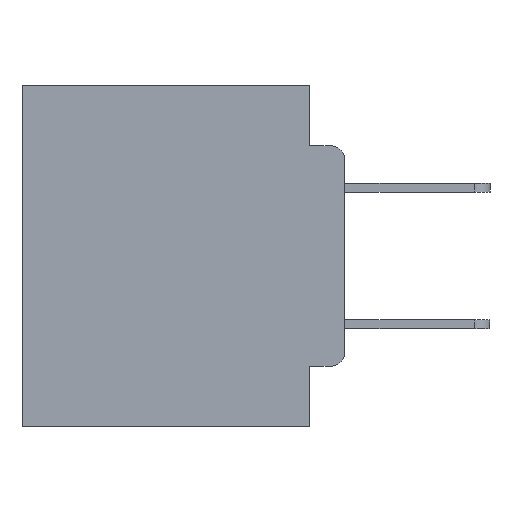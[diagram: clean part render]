
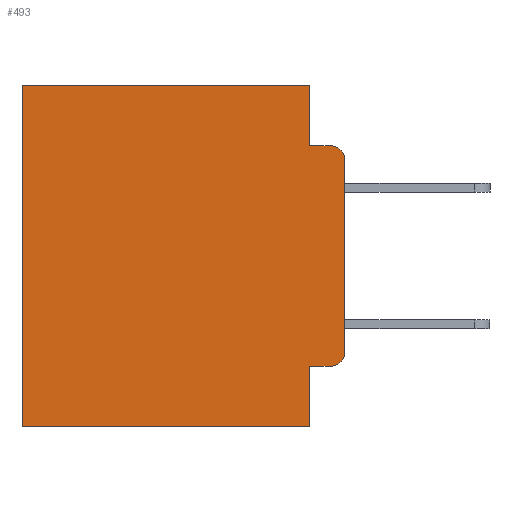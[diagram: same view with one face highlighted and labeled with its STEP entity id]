
A CAD part, left-side view. The second image highlights one B-rep face of the part: STEP entity #493.
In plain terms, the highlighted planar face has unit normal (-1, 0, 0).
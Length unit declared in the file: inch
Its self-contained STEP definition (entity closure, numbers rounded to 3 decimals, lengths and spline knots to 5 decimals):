
#359 = VERTEX_POINT ( 'NONE', #24154 ) ;
#385 = EDGE_CURVE ( 'NONE', #1423, #24243, #5660, .T. ) ;
#493 = ADVANCED_FACE ( 'NONE', ( #2331 ), #21207, .F. ) ;
#886 = DIRECTION ( 'NONE',  ( 0., 0., -1. ) ) ;
#1332 = DIRECTION ( 'NONE',  ( -1., 0., 0. ) ) ;
#1423 = VERTEX_POINT ( 'NONE', #10950 ) ;
#1480 = DIRECTION ( 'NONE',  ( 0., 1., 0. ) ) ;
#1768 = CARTESIAN_POINT ( 'NONE',  ( 0.298, 0.051, 0. ) ) ;
#2240 = EDGE_CURVE ( 'NONE', #6536, #1423, #15348, .T. ) ;
#2331 = FACE_OUTER_BOUND ( 'NONE', #25447, .T. ) ;
#2547 = VECTOR ( 'NONE', #12413, 39.37008 ) ;
#2775 = DIRECTION ( 'NONE',  ( -1., 0., 0. ) ) ;
#2864 = VERTEX_POINT ( 'NONE', #21448 ) ;
#3146 = CIRCLE ( 'NONE', #5837, 0.02 ) ;
#3339 = ORIENTED_EDGE ( 'NONE', *, *, #2240, .F. ) ;
#3368 = CARTESIAN_POINT ( 'NONE',  ( 0.298, 0.051, -0.4115 ) ) ;
#3389 = CARTESIAN_POINT ( 'NONE',  ( 0.298, 0., 0. ) ) ;
#4218 = VERTEX_POINT ( 'NONE', #23876 ) ;
#4588 = ORIENTED_EDGE ( 'NONE', *, *, #19473, .F. ) ;
#5006 = LINE ( 'NONE', #6739, #26039 ) ;
#5660 = LINE ( 'NONE', #9719, #10527 ) ;
#5837 = AXIS2_PLACEMENT_3D ( 'NONE', #15330, #2775, #17415 ) ;
#5911 = ORIENTED_EDGE ( 'NONE', *, *, #385, .F. ) ;
#6536 = VERTEX_POINT ( 'NONE', #11594 ) ;
#6739 = CARTESIAN_POINT ( 'NONE',  ( 0.298, 0.473, 0. ) ) ;
#6945 = ORIENTED_EDGE ( 'NONE', *, *, #20773, .T. ) ;
#7207 = DIRECTION ( 'NONE',  ( 1., 0., 0. ) ) ;
#7208 = ORIENTED_EDGE ( 'NONE', *, *, #10673, .T. ) ;
#7317 = CARTESIAN_POINT ( 'NONE',  ( 0.298, 0.051, 0. ) ) ;
#7324 = EDGE_CURVE ( 'NONE', #13859, #15356, #12450, .T. ) ;
#8261 = ORIENTED_EDGE ( 'NONE', *, *, #23401, .T. ) ;
#9406 = CARTESIAN_POINT ( 'NONE',  ( 0.298, 0.473, 0. ) ) ;
#9719 = CARTESIAN_POINT ( 'NONE',  ( 0.298, 0., -0.5 ) ) ;
#10087 = CARTESIAN_POINT ( 'NONE',  ( 0.298, 0.051, -0.0885 ) ) ;
#10432 = LINE ( 'NONE', #3368, #15362 ) ;
#10457 = LINE ( 'NONE', #7317, #20096 ) ;
#10527 = VECTOR ( 'NONE', #21945, 39.37008 ) ;
#10673 = EDGE_CURVE ( 'NONE', #359, #20845, #3146, .T. ) ;
#10950 = CARTESIAN_POINT ( 'NONE',  ( 0.298, 0.051, -0.5 ) ) ;
#11197 = EDGE_CURVE ( 'NONE', #4218, #20845, #23631, .T. ) ;
#11594 = CARTESIAN_POINT ( 'NONE',  ( 0.298, 0.051, -0.4115 ) ) ;
#12413 = DIRECTION ( 'NONE',  ( 0., -1., 0. ) ) ;
#12450 = LINE ( 'NONE', #3389, #22564 ) ;
#12937 = VECTOR ( 'NONE', #17035, 39.37008 ) ;
#13859 = VERTEX_POINT ( 'NONE', #1768 ) ;
#13948 = CARTESIAN_POINT ( 'NONE',  ( 0.298, 0.02, -0.1085 ) ) ;
#14278 = DIRECTION ( 'NONE',  ( 0., 0., -1. ) ) ;
#15330 = CARTESIAN_POINT ( 'NONE',  ( 0.298, 0.02, -0.3915 ) ) ;
#15348 = LINE ( 'NONE', #23893, #20662 ) ;
#15356 = VERTEX_POINT ( 'NONE', #9406 ) ;
#15362 = VECTOR ( 'NONE', #21883, 39.37008 ) ;
#16054 = DIRECTION ( 'NONE',  ( 0., 0., -1. ) ) ;
#16336 = CARTESIAN_POINT ( 'NONE',  ( 0.298, 0., -0.3915 ) ) ;
#16563 = DIRECTION ( 'NONE',  ( 0., 0., -1. ) ) ;
#17035 = DIRECTION ( 'NONE',  ( 0., 0., -1. ) ) ;
#17098 = CARTESIAN_POINT ( 'NONE',  ( 0.298, 0., 0. ) ) ;
#17415 = DIRECTION ( 'NONE',  ( 0., 0., -1. ) ) ;
#18250 = CARTESIAN_POINT ( 'NONE',  ( 0.298, 0.473, -0.5 ) ) ;
#18641 = ORIENTED_EDGE ( 'NONE', *, *, #24714, .F. ) ;
#19473 = EDGE_CURVE ( 'NONE', #20274, #2864, #23109, .T. ) ;
#20096 = VECTOR ( 'NONE', #886, 39.37008 ) ;
#20274 = VERTEX_POINT ( 'NONE', #10087 ) ;
#20394 = ORIENTED_EDGE ( 'NONE', *, *, #11197, .F. ) ;
#20662 = VECTOR ( 'NONE', #14278, 39.37008 ) ;
#20773 = EDGE_CURVE ( 'NONE', #4218, #2864, #24894, .T. ) ;
#20845 = VERTEX_POINT ( 'NONE', #16336 ) ;
#20976 = AXIS2_PLACEMENT_3D ( 'NONE', #13948, #1332, #16054 ) ;
#21207 = PLANE ( 'NONE',  #23602 ) ;
#21448 = CARTESIAN_POINT ( 'NONE',  ( 0.298, 0.02, -0.0885 ) ) ;
#21619 = ORIENTED_EDGE ( 'NONE', *, *, #7324, .T. ) ;
#21883 = DIRECTION ( 'NONE',  ( 0., -1., 0. ) ) ;
#21945 = DIRECTION ( 'NONE',  ( 0., 1., 0. ) ) ;
#22564 = VECTOR ( 'NONE', #1480, 39.37008 ) ;
#22841 = ORIENTED_EDGE ( 'NONE', *, *, #26074, .T. ) ;
#22863 = CARTESIAN_POINT ( 'NONE',  ( 0.298, 0., 0. ) ) ;
#23072 = DIRECTION ( 'NONE',  ( 0., 0., -1. ) ) ;
#23109 = LINE ( 'NONE', #24461, #2547 ) ;
#23401 = EDGE_CURVE ( 'NONE', #15356, #24243, #5006, .T. ) ;
#23602 = AXIS2_PLACEMENT_3D ( 'NONE', #17098, #7207, #16563 ) ;
#23631 = LINE ( 'NONE', #22863, #12937 ) ;
#23876 = CARTESIAN_POINT ( 'NONE',  ( 0.298, 0., -0.1085 ) ) ;
#23893 = CARTESIAN_POINT ( 'NONE',  ( 0.298, 0.051, 0. ) ) ;
#24154 = CARTESIAN_POINT ( 'NONE',  ( 0.298, 0.02, -0.4115 ) ) ;
#24243 = VERTEX_POINT ( 'NONE', #18250 ) ;
#24461 = CARTESIAN_POINT ( 'NONE',  ( 0.298, 0.051, -0.0885 ) ) ;
#24714 = EDGE_CURVE ( 'NONE', #13859, #20274, #10457, .T. ) ;
#24894 = CIRCLE ( 'NONE', #20976, 0.02 ) ;
#25447 = EDGE_LOOP ( 'NONE', ( #20394, #6945, #4588, #18641, #21619, #8261, #5911, #3339, #22841, #7208 ) ) ;
#26039 = VECTOR ( 'NONE', #23072, 39.37008 ) ;
#26074 = EDGE_CURVE ( 'NONE', #6536, #359, #10432, .T. ) ;
